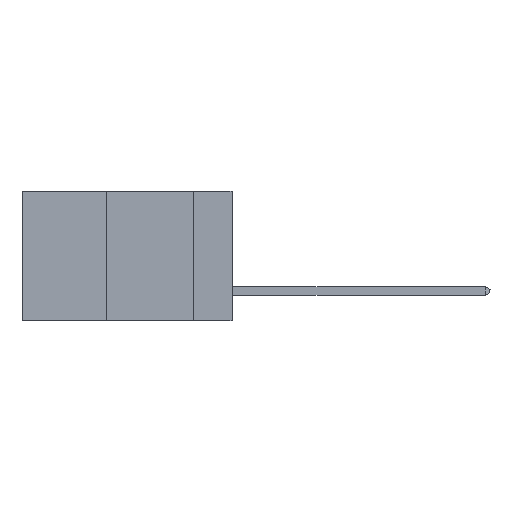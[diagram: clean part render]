
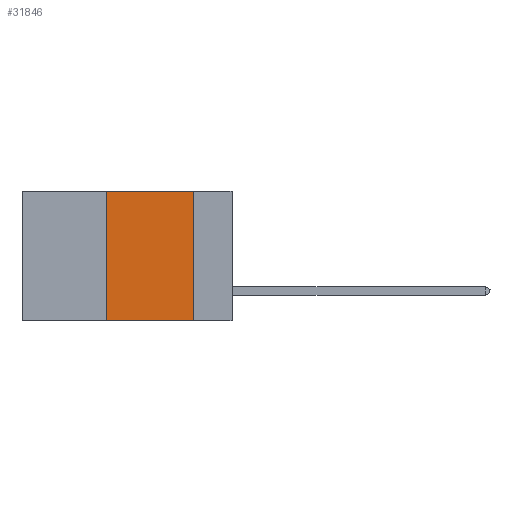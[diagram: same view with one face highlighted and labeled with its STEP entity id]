
A CAD part, left-side view. The second image highlights one B-rep face of the part: STEP entity #31846.
In plain terms, the highlighted planar face has unit normal (-1, 0, 0).
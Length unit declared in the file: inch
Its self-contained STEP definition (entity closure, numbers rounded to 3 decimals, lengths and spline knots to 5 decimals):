
#2791 = CARTESIAN_POINT ( 'NONE',  ( 0., 0.36, 0. ) ) ;
#4887 = DIRECTION ( 'NONE',  ( 0., -1., 0. ) ) ;
#4921 = VERTEX_POINT ( 'NONE', #11571 ) ;
#7299 = EDGE_LOOP ( 'NONE', ( #34442, #36871, #26122, #26639 ) ) ;
#7560 = EDGE_CURVE ( 'NONE', #14700, #4921, #36028, .T. ) ;
#7791 = CARTESIAN_POINT ( 'NONE',  ( 0., 0.6, 0. ) ) ;
#8665 = DIRECTION ( 'NONE',  ( 1., 0., 0. ) ) ;
#10724 = VERTEX_POINT ( 'NONE', #26432 ) ;
#11571 = CARTESIAN_POINT ( 'NONE',  ( 0., 0.11, 0. ) ) ;
#12974 = FACE_OUTER_BOUND ( 'NONE', #7299, .T. ) ;
#14700 = VERTEX_POINT ( 'NONE', #2791 ) ;
#14856 = PLANE ( 'NONE',  #34357 ) ;
#17738 = CARTESIAN_POINT ( 'NONE',  ( 0., 0.11, 0. ) ) ;
#18469 = CARTESIAN_POINT ( 'NONE',  ( 0., 0.11, -0.37 ) ) ;
#19330 = DIRECTION ( 'NONE',  ( 0., 0., 1. ) ) ;
#19512 = CARTESIAN_POINT ( 'NONE',  ( 0., 0.6, -0.37 ) ) ;
#20342 = VERTEX_POINT ( 'NONE', #18469 ) ;
#21145 = LINE ( 'NONE', #22361, #25600 ) ;
#22361 = CARTESIAN_POINT ( 'NONE',  ( 0., 0.36, 0. ) ) ;
#24830 = DIRECTION ( 'NONE',  ( 0., 0., -1. ) ) ;
#25600 = VECTOR ( 'NONE', #19330, 39.37008 ) ;
#26122 = ORIENTED_EDGE ( 'NONE', *, *, #29023, .F. ) ;
#26143 = VECTOR ( 'NONE', #38871, 39.37008 ) ;
#26432 = CARTESIAN_POINT ( 'NONE',  ( 0., 0.36, -0.37 ) ) ;
#26639 = ORIENTED_EDGE ( 'NONE', *, *, #36223, .T. ) ;
#27139 = LINE ( 'NONE', #19512, #26143 ) ;
#29023 = EDGE_CURVE ( 'NONE', #10724, #14700, #21145, .T. ) ;
#29549 = LINE ( 'NONE', #17738, #40485 ) ;
#29611 = EDGE_CURVE ( 'NONE', #4921, #20342, #29549, .T. ) ;
#30787 = DIRECTION ( 'NONE',  ( 0., 0., -1. ) ) ;
#31846 = ADVANCED_FACE ( 'NONE', ( #12974 ), #14856, .F. ) ;
#34357 = AXIS2_PLACEMENT_3D ( 'NONE', #40381, #8665, #30787 ) ;
#34442 = ORIENTED_EDGE ( 'NONE', *, *, #29611, .F. ) ;
#35013 = VECTOR ( 'NONE', #4887, 39.37008 ) ;
#36028 = LINE ( 'NONE', #7791, #35013 ) ;
#36223 = EDGE_CURVE ( 'NONE', #10724, #20342, #27139, .T. ) ;
#36871 = ORIENTED_EDGE ( 'NONE', *, *, #7560, .F. ) ;
#38871 = DIRECTION ( 'NONE',  ( 0., -1., 0. ) ) ;
#40381 = CARTESIAN_POINT ( 'NONE',  ( 0., 0.6, 0. ) ) ;
#40485 = VECTOR ( 'NONE', #24830, 39.37008 ) ;
